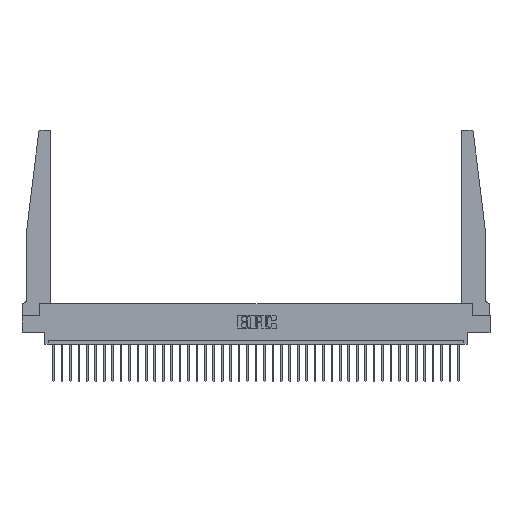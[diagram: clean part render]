
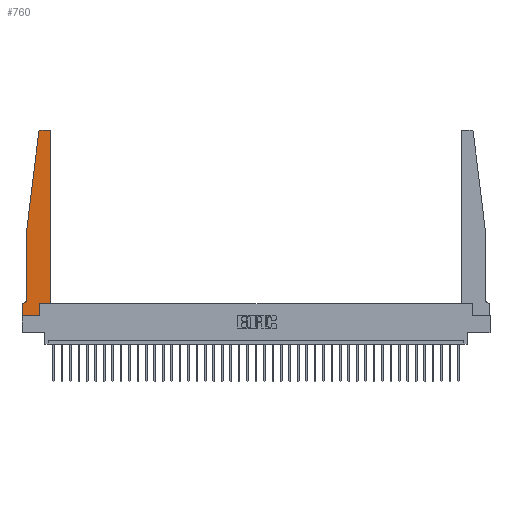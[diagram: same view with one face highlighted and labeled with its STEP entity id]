
A CAD part, top view. The second image highlights one B-rep face of the part: STEP entity #760.
In plain terms, the highlighted planar face has unit normal (0, 0, 1).
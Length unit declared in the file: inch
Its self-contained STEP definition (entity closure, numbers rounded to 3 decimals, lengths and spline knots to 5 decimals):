
#311 = LINE ( 'NONE', #10506, #20644 ) ;
#314 = CARTESIAN_POINT ( 'NONE',  ( 0.425, 0.18, 0.37 ) ) ;
#760 = ADVANCED_FACE ( 'NONE', ( #24253 ), #24656, .T. ) ;
#951 = CARTESIAN_POINT ( 'NONE',  ( 0.2605, 0.18, 0.37 ) ) ;
#971 = EDGE_CURVE ( 'NONE', #13155, #6389, #12587, .T. ) ;
#1870 = CARTESIAN_POINT ( 'NONE',  ( 0.2605, 0.18, 0.37 ) ) ;
#3147 = CARTESIAN_POINT ( 'NONE',  ( 0.065, 1.25, 0.37 ) ) ;
#3186 = LINE ( 'NONE', #1870, #29786 ) ;
#3292 = EDGE_CURVE ( 'NONE', #31083, #12162, #29059, .T. ) ;
#3377 = LINE ( 'NONE', #17215, #31228 ) ;
#4336 = VECTOR ( 'NONE', #6823, 39.37008 ) ;
#4584 = EDGE_LOOP ( 'NONE', ( #21970, #17059, #10135, #28603, #8726, #17913, #34246, #13670, #13141, #32807, #5129, #26112 ) ) ;
#5129 = ORIENTED_EDGE ( 'NONE', *, *, #24408, .T. ) ;
#5767 = CARTESIAN_POINT ( 'NONE',  ( 0.25, 2.75, 0.37 ) ) ;
#5935 = CIRCLE ( 'NONE', #6921, 0.05 ) ;
#6085 = CARTESIAN_POINT ( 'NONE',  ( 0.2605, 0., 0.37 ) ) ;
#6389 = VERTEX_POINT ( 'NONE', #13682 ) ;
#6551 = DIRECTION ( 'NONE',  ( 0., 0., 1. ) ) ;
#6823 = DIRECTION ( 'NONE',  ( 1., 0., 0. ) ) ;
#6921 = AXIS2_PLACEMENT_3D ( 'NONE', #32441, #22922, #9917 ) ;
#7475 = VECTOR ( 'NONE', #34093, 39.37008 ) ;
#7596 = CARTESIAN_POINT ( 'NONE',  ( 0.24675, 2.72367, 0.37 ) ) ;
#8726 = ORIENTED_EDGE ( 'NONE', *, *, #22506, .T. ) ;
#8857 = VECTOR ( 'NONE', #29116, 39.37008 ) ;
#9087 = EDGE_CURVE ( 'NONE', #30668, #13122, #15787, .T. ) ;
#9917 = DIRECTION ( 'NONE',  ( -1., 0., 0. ) ) ;
#9972 = DIRECTION ( 'NONE',  ( 0., 1., 0. ) ) ;
#10041 = VERTEX_POINT ( 'NONE', #7596 ) ;
#10135 = ORIENTED_EDGE ( 'NONE', *, *, #20174, .T. ) ;
#10247 = EDGE_CURVE ( 'NONE', #25026, #10041, #33582, .T. ) ;
#10506 = CARTESIAN_POINT ( 'NONE',  ( 0.065, 1.25, 0.37 ) ) ;
#10789 = CARTESIAN_POINT ( 'NONE',  ( 0.015, 0.1875, 0.37 ) ) ;
#11335 = EDGE_CURVE ( 'NONE', #30377, #31083, #3186, .T. ) ;
#11684 = CARTESIAN_POINT ( 'NONE',  ( 0.395, 2.72, 0.37 ) ) ;
#12162 = VERTEX_POINT ( 'NONE', #19606 ) ;
#12502 = VECTOR ( 'NONE', #16104, 39.37008 ) ;
#12587 = LINE ( 'NONE', #21114, #8857 ) ;
#12660 = LINE ( 'NONE', #30987, #4336 ) ;
#13122 = VERTEX_POINT ( 'NONE', #24382 ) ;
#13141 = ORIENTED_EDGE ( 'NONE', *, *, #11335, .T. ) ;
#13155 = VERTEX_POINT ( 'NONE', #3147 ) ;
#13670 = ORIENTED_EDGE ( 'NONE', *, *, #17096, .T. ) ;
#13671 = CARTESIAN_POINT ( 'NONE',  ( 0.27653, 2.75, 0.37 ) ) ;
#13682 = CARTESIAN_POINT ( 'NONE',  ( 0.065, 0.2375, 0.37 ) ) ;
#15607 = DIRECTION ( 'NONE',  ( -0.122, -0.992, 0. ) ) ;
#15672 = VERTEX_POINT ( 'NONE', #10789 ) ;
#15787 = LINE ( 'NONE', #23408, #7475 ) ;
#16104 = DIRECTION ( 'NONE',  ( -1., 0., 0. ) ) ;
#17059 = ORIENTED_EDGE ( 'NONE', *, *, #10247, .T. ) ;
#17096 = EDGE_CURVE ( 'NONE', #13122, #30377, #12660, .T. ) ;
#17215 = CARTESIAN_POINT ( 'NONE',  ( 0.065, 0.1875, 0.37 ) ) ;
#17913 = ORIENTED_EDGE ( 'NONE', *, *, #32592, .T. ) ;
#18167 = DIRECTION ( 'NONE',  ( 1., 0., 0. ) ) ;
#19104 = DIRECTION ( 'NONE',  ( 1., 0., 0. ) ) ;
#19334 = DIRECTION ( 'NONE',  ( -1., 0., 0. ) ) ;
#19557 = VECTOR ( 'NONE', #33971, 39.37008 ) ;
#19606 = CARTESIAN_POINT ( 'NONE',  ( 0.425, 0.18, 0.37 ) ) ;
#20174 = EDGE_CURVE ( 'NONE', #10041, #13155, #311, .T. ) ;
#20644 = VECTOR ( 'NONE', #15607, 39.37008 ) ;
#20745 = VECTOR ( 'NONE', #26873, 39.37008 ) ;
#21114 = CARTESIAN_POINT ( 'NONE',  ( 0.065, 1.25, 0.37 ) ) ;
#21967 = CARTESIAN_POINT ( 'NONE',  ( 0., 0.1875, 0.37 ) ) ;
#21970 = ORIENTED_EDGE ( 'NONE', *, *, #33523, .T. ) ;
#22113 = VERTEX_POINT ( 'NONE', #22502 ) ;
#22502 = CARTESIAN_POINT ( 'NONE',  ( 0.425, 2.72, 0.37 ) ) ;
#22506 = EDGE_CURVE ( 'NONE', #6389, #15672, #5935, .T. ) ;
#22922 = DIRECTION ( 'NONE',  ( 0., 0., -1. ) ) ;
#23244 = CARTESIAN_POINT ( 'NONE',  ( 0., 0.1875, 0.37 ) ) ;
#23408 = CARTESIAN_POINT ( 'NONE',  ( 0., 0., 0.37 ) ) ;
#23527 = AXIS2_PLACEMENT_3D ( 'NONE', #28462, #23597, #18167 ) ;
#23597 = DIRECTION ( 'NONE',  ( 0., 0., 1. ) ) ;
#24253 = FACE_OUTER_BOUND ( 'NONE', #4584, .T. ) ;
#24382 = CARTESIAN_POINT ( 'NONE',  ( 0., 0., 0.37 ) ) ;
#24408 = EDGE_CURVE ( 'NONE', #12162, #22113, #26587, .T. ) ;
#24445 = EDGE_CURVE ( 'NONE', #22113, #27428, #26176, .T. ) ;
#24656 = PLANE ( 'NONE',  #30316 ) ;
#25026 = VERTEX_POINT ( 'NONE', #13671 ) ;
#25069 = CARTESIAN_POINT ( 'NONE',  ( 0.425, 0.18, 0.37 ) ) ;
#26112 = ORIENTED_EDGE ( 'NONE', *, *, #24445, .T. ) ;
#26176 = CIRCLE ( 'NONE', #26285, 0.03 ) ;
#26285 = AXIS2_PLACEMENT_3D ( 'NONE', #11684, #6551, #30273 ) ;
#26587 = LINE ( 'NONE', #25069, #19557 ) ;
#26873 = DIRECTION ( 'NONE',  ( 1., 0., 0. ) ) ;
#27428 = VERTEX_POINT ( 'NONE', #28524 ) ;
#28462 = CARTESIAN_POINT ( 'NONE',  ( 0.27653, 2.72, 0.37 ) ) ;
#28524 = CARTESIAN_POINT ( 'NONE',  ( 0.395, 2.75, 0.37 ) ) ;
#28603 = ORIENTED_EDGE ( 'NONE', *, *, #971, .T. ) ;
#29059 = LINE ( 'NONE', #314, #20745 ) ;
#29116 = DIRECTION ( 'NONE',  ( 0., -1., 0. ) ) ;
#29786 = VECTOR ( 'NONE', #9972, 39.37008 ) ;
#30273 = DIRECTION ( 'NONE',  ( 1., 0., 0. ) ) ;
#30316 = AXIS2_PLACEMENT_3D ( 'NONE', #21967, #32191, #19104 ) ;
#30377 = VERTEX_POINT ( 'NONE', #6085 ) ;
#30668 = VERTEX_POINT ( 'NONE', #23244 ) ;
#30987 = CARTESIAN_POINT ( 'NONE',  ( 0., 0., 0.37 ) ) ;
#31083 = VERTEX_POINT ( 'NONE', #951 ) ;
#31228 = VECTOR ( 'NONE', #19334, 39.37008 ) ;
#32191 = DIRECTION ( 'NONE',  ( 0., 0., 1. ) ) ;
#32441 = CARTESIAN_POINT ( 'NONE',  ( 0.015, 0.2375, 0.37 ) ) ;
#32592 = EDGE_CURVE ( 'NONE', #15672, #30668, #3377, .T. ) ;
#32807 = ORIENTED_EDGE ( 'NONE', *, *, #3292, .T. ) ;
#33523 = EDGE_CURVE ( 'NONE', #27428, #25026, #33681, .T. ) ;
#33582 = CIRCLE ( 'NONE', #23527, 0.03 ) ;
#33681 = LINE ( 'NONE', #5767, #12502 ) ;
#33971 = DIRECTION ( 'NONE',  ( 0., 1., 0. ) ) ;
#34093 = DIRECTION ( 'NONE',  ( 0., -1., 0. ) ) ;
#34246 = ORIENTED_EDGE ( 'NONE', *, *, #9087, .T. ) ;
